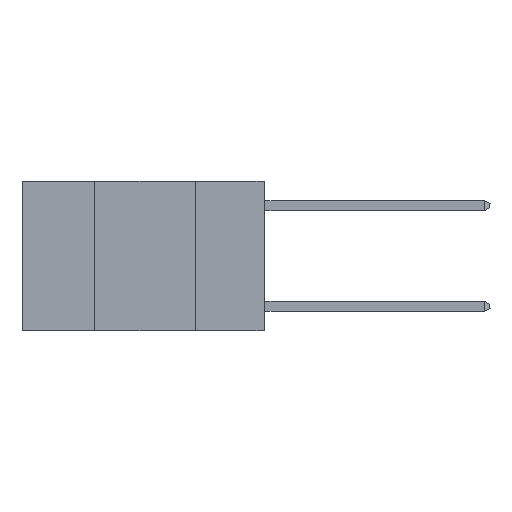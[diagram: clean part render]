
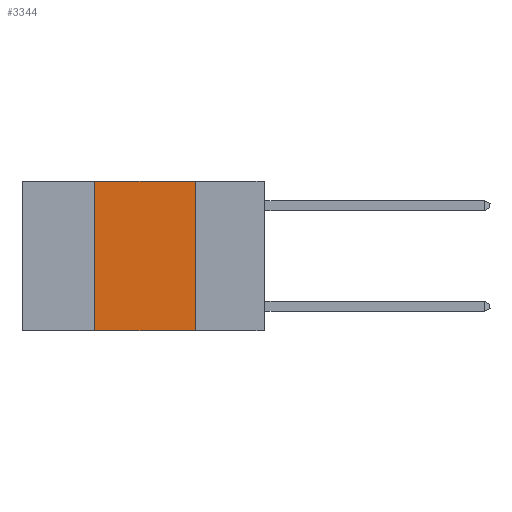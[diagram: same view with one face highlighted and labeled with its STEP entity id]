
A CAD part, left-side view. The second image highlights one B-rep face of the part: STEP entity #3344.
In plain terms, the highlighted planar face has unit normal (-1, 0, 0).
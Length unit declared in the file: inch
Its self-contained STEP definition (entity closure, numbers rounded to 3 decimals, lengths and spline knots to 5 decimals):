
#620 = ORIENTED_EDGE ( 'NONE', *, *, #1964, .F. ) ;
#1233 = LINE ( 'NONE', #5921, #7302 ) ;
#1284 = PLANE ( 'NONE',  #6845 ) ;
#1510 = LINE ( 'NONE', #6167, #6962 ) ;
#1964 = EDGE_CURVE ( 'NONE', #6373, #5289, #6861, .T. ) ;
#2214 = DIRECTION ( 'NONE',  ( 0., 0., 1. ) ) ;
#2961 = CARTESIAN_POINT ( 'NONE',  ( 0., 0.42, 0. ) ) ;
#3006 = FACE_OUTER_BOUND ( 'NONE', #5980, .T. ) ;
#3126 = CARTESIAN_POINT ( 'NONE',  ( 0., 0.42, -0.37 ) ) ;
#3260 = ORIENTED_EDGE ( 'NONE', *, *, #6379, .F. ) ;
#3344 = ADVANCED_FACE ( 'NONE', ( #3006 ), #1284, .F. ) ;
#3429 = ORIENTED_EDGE ( 'NONE', *, *, #6225, .T. ) ;
#3885 = VECTOR ( 'NONE', #6086, 39.37008 ) ;
#4005 = VERTEX_POINT ( 'NONE', #4086 ) ;
#4086 = CARTESIAN_POINT ( 'NONE',  ( 0., 0.42, 0. ) ) ;
#4415 = DIRECTION ( 'NONE',  ( 1., 0., 0. ) ) ;
#4666 = DIRECTION ( 'NONE',  ( 0., -1., 0. ) ) ;
#5084 = EDGE_CURVE ( 'NONE', #10307, #4005, #10100, .T. ) ;
#5148 = DIRECTION ( 'NONE',  ( 0., -1., 0. ) ) ;
#5289 = VERTEX_POINT ( 'NONE', #6620 ) ;
#5520 = CARTESIAN_POINT ( 'NONE',  ( 0., 0.17, 0. ) ) ;
#5921 = CARTESIAN_POINT ( 'NONE',  ( 0., 0.6, -0.37 ) ) ;
#5973 = CARTESIAN_POINT ( 'NONE',  ( 0., 0.6, 0. ) ) ;
#5980 = EDGE_LOOP ( 'NONE', ( #620, #3260, #9567, #3429 ) ) ;
#6086 = DIRECTION ( 'NONE',  ( 0., 0., -1. ) ) ;
#6167 = CARTESIAN_POINT ( 'NONE',  ( 0., 0.6, 0. ) ) ;
#6225 = EDGE_CURVE ( 'NONE', #10307, #5289, #1233, .T. ) ;
#6373 = VERTEX_POINT ( 'NONE', #5520 ) ;
#6379 = EDGE_CURVE ( 'NONE', #4005, #6373, #1510, .T. ) ;
#6620 = CARTESIAN_POINT ( 'NONE',  ( 0., 0.17, -0.37 ) ) ;
#6845 = AXIS2_PLACEMENT_3D ( 'NONE', #5973, #4415, #7732 ) ;
#6861 = LINE ( 'NONE', #10068, #3885 ) ;
#6962 = VECTOR ( 'NONE', #4666, 39.37008 ) ;
#7302 = VECTOR ( 'NONE', #5148, 39.37008 ) ;
#7732 = DIRECTION ( 'NONE',  ( 0., 0., -1. ) ) ;
#9567 = ORIENTED_EDGE ( 'NONE', *, *, #5084, .F. ) ;
#9693 = VECTOR ( 'NONE', #2214, 39.37008 ) ;
#10068 = CARTESIAN_POINT ( 'NONE',  ( 0., 0.17, 0. ) ) ;
#10100 = LINE ( 'NONE', #2961, #9693 ) ;
#10307 = VERTEX_POINT ( 'NONE', #3126 ) ;
